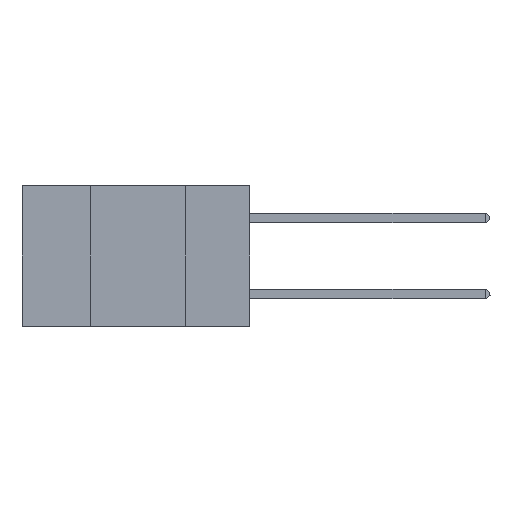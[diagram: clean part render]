
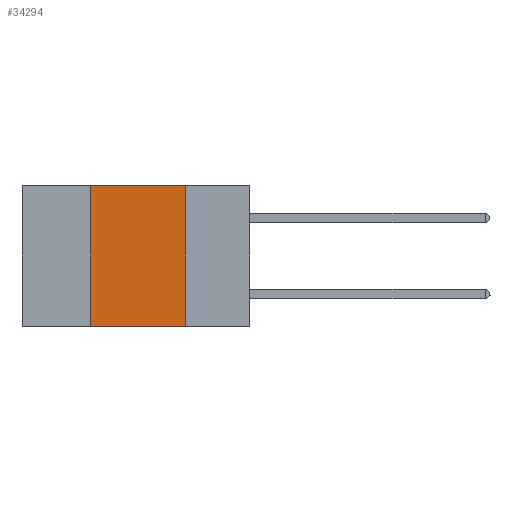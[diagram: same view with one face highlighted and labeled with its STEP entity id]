
A CAD part, left-side view. The second image highlights one B-rep face of the part: STEP entity #34294.
In plain terms, the highlighted planar face has unit normal (-1, 0, 0).
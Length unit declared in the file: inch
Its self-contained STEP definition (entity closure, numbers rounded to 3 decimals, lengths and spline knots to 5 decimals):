
#807 = LINE ( 'NONE', #1211, #28148 ) ;
#1211 = CARTESIAN_POINT ( 'NONE',  ( 0., 0.42, 0. ) ) ;
#1748 = LINE ( 'NONE', #2571, #19185 ) ;
#2459 = DIRECTION ( 'NONE',  ( 0., -1., 0. ) ) ;
#2571 = CARTESIAN_POINT ( 'NONE',  ( 0., 0.6, -0.37 ) ) ;
#5021 = ORIENTED_EDGE ( 'NONE', *, *, #22080, .F. ) ;
#6277 = ORIENTED_EDGE ( 'NONE', *, *, #30781, .F. ) ;
#6386 = CARTESIAN_POINT ( 'NONE',  ( 0., 0.6, 0. ) ) ;
#6721 = DIRECTION ( 'NONE',  ( 0., 0., -1. ) ) ;
#8458 = FACE_OUTER_BOUND ( 'NONE', #18627, .T. ) ;
#9055 = CARTESIAN_POINT ( 'NONE',  ( 0., 0.6, 0. ) ) ;
#9941 = AXIS2_PLACEMENT_3D ( 'NONE', #6386, #16924, #6721 ) ;
#10888 = VECTOR ( 'NONE', #25136, 39.37008 ) ;
#12231 = LINE ( 'NONE', #32062, #26712 ) ;
#14742 = CARTESIAN_POINT ( 'NONE',  ( 0., 0.42, 0. ) ) ;
#16924 = DIRECTION ( 'NONE',  ( 1., 0., 0. ) ) ;
#18627 = EDGE_LOOP ( 'NONE', ( #31523, #6277, #5021, #20619 ) ) ;
#18665 = CARTESIAN_POINT ( 'NONE',  ( 0., 0.17, 0. ) ) ;
#18753 = VERTEX_POINT ( 'NONE', #14742 ) ;
#19185 = VECTOR ( 'NONE', #2459, 39.37008 ) ;
#20462 = EDGE_CURVE ( 'NONE', #21040, #28203, #1748, .T. ) ;
#20619 = ORIENTED_EDGE ( 'NONE', *, *, #20462, .T. ) ;
#21040 = VERTEX_POINT ( 'NONE', #28698 ) ;
#22080 = EDGE_CURVE ( 'NONE', #21040, #18753, #807, .T. ) ;
#22628 = DIRECTION ( 'NONE',  ( 0., 0., 1. ) ) ;
#25136 = DIRECTION ( 'NONE',  ( 0., -1., 0. ) ) ;
#26595 = LINE ( 'NONE', #9055, #10888 ) ;
#26712 = VECTOR ( 'NONE', #26861, 39.37008 ) ;
#26861 = DIRECTION ( 'NONE',  ( 0., 0., -1. ) ) ;
#28148 = VECTOR ( 'NONE', #22628, 39.37008 ) ;
#28203 = VERTEX_POINT ( 'NONE', #31958 ) ;
#28698 = CARTESIAN_POINT ( 'NONE',  ( 0., 0.42, -0.37 ) ) ;
#30781 = EDGE_CURVE ( 'NONE', #18753, #33999, #26595, .T. ) ;
#31523 = ORIENTED_EDGE ( 'NONE', *, *, #33975, .F. ) ;
#31958 = CARTESIAN_POINT ( 'NONE',  ( 0., 0.17, -0.37 ) ) ;
#32062 = CARTESIAN_POINT ( 'NONE',  ( 0., 0.17, 0. ) ) ;
#33087 = PLANE ( 'NONE',  #9941 ) ;
#33975 = EDGE_CURVE ( 'NONE', #33999, #28203, #12231, .T. ) ;
#33999 = VERTEX_POINT ( 'NONE', #18665 ) ;
#34294 = ADVANCED_FACE ( 'NONE', ( #8458 ), #33087, .F. ) ;
